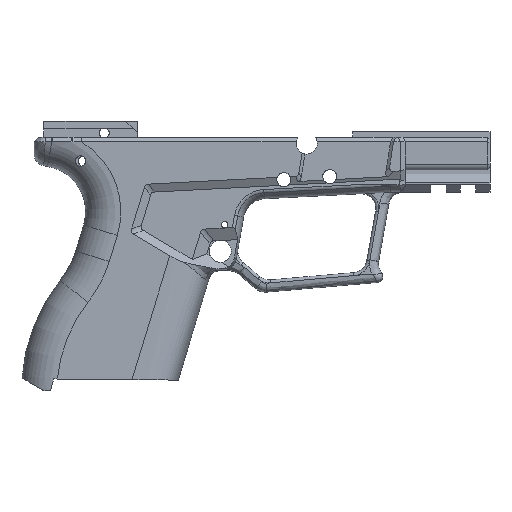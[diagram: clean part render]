
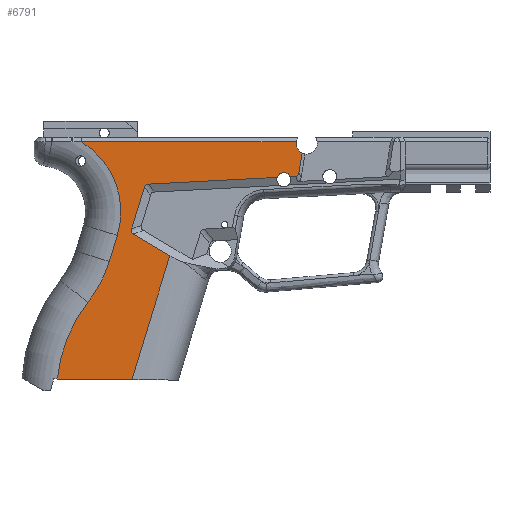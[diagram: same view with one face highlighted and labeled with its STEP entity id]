
A CAD part, left-side view. The second image highlights one B-rep face of the part: STEP entity #6791.
In plain terms, the highlighted planar face has unit normal (-1, 0, 0).
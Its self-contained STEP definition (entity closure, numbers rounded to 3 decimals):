
#60=ELLIPSE('',#6874,4.209,2.);
#64=ELLIPSE('',#6880,7.017,3.);
#66=ELLIPSE('',#6884,7.254,3.);
#545=PLANE('',#7359);
#892=FACE_OUTER_BOUND('',#1259,.T.);
#1259=EDGE_LOOP('',(#6368,#6369,#6370,#6371,#6372,#6373,#6374,#6375,#6376,
#6377,#6378,#6379,#6380,#6381,#6382,#6383,#6384,#6385));
#1333=CIRCLE('',#7027,2.4);
#1336=CIRCLE('',#7032,3.625);
#1445=CIRCLE('',#7334,48.221);
#1452=CIRCLE('',#7360,27.5);
#1453=CIRCLE('',#7361,42.);
#1534=LINE('',#9499,#2189);
#1575=LINE('',#9775,#2230);
#1579=LINE('',#9790,#2234);
#1584=LINE('',#9803,#2239);
#1587=LINE('',#9812,#2242);
#1589=LINE('',#9842,#2244);
#2095=LINE('',#15264,#2750);
#2109=LINE('',#15326,#2764);
#2110=LINE('',#15331,#2765);
#2111=LINE('',#15333,#2766);
#2189=VECTOR('',#7510,1000.);
#2230=VECTOR('',#7611,10.);
#2234=VECTOR('',#7625,10.);
#2239=VECTOR('',#7638,10.);
#2242=VECTOR('',#7649,10.);
#2244=VECTOR('',#7661,10.);
#2750=VECTOR('',#9075,10.);
#2764=VECTOR('',#9117,10.);
#2765=VECTOR('',#9122,10.);
#2766=VECTOR('',#9125,10.);
#2841=VERTEX_POINT('',#9497);
#2842=VERTEX_POINT('',#9498);
#2886=VERTEX_POINT('',#9772);
#2887=VERTEX_POINT('',#9774);
#2888=VERTEX_POINT('',#9778);
#2892=VERTEX_POINT('',#9787);
#2893=VERTEX_POINT('',#9789);
#2895=VERTEX_POINT('',#9795);
#2897=VERTEX_POINT('',#9800);
#2899=VERTEX_POINT('',#9807);
#2902=VERTEX_POINT('',#9836);
#3069=VERTEX_POINT('',#10879);
#3376=VERTEX_POINT('',#15017);
#3385=VERTEX_POINT('',#15198);
#3390=VERTEX_POINT('',#15231);
#3399=VERTEX_POINT('',#15262);
#3408=VERTEX_POINT('',#15328);
#3409=VERTEX_POINT('',#15330);
#3504=EDGE_CURVE('',#2841,#2842,#1534,.T.);
#3565=EDGE_CURVE('',#2887,#2886,#1575,.T.);
#3567=EDGE_CURVE('',#2887,#2888,#60,.T.);
#3572=EDGE_CURVE('',#2893,#2892,#1579,.T.);
#3575=EDGE_CURVE('',#2893,#2895,#64,.T.);
#3579=EDGE_CURVE('',#2897,#2895,#1584,.T.);
#3581=EDGE_CURVE('',#2897,#2899,#66,.T.);
#3584=EDGE_CURVE('',#2841,#2899,#1587,.T.);
#3592=EDGE_CURVE('',#2902,#2888,#1589,.T.);
#3823=EDGE_CURVE('',#2892,#2902,#1333,.F.);
#3830=EDGE_CURVE('',#2886,#3069,#1336,.T.);
#4375=EDGE_CURVE('',#3390,#3385,#1445,.T.);
#4391=EDGE_CURVE('',#3390,#3399,#2095,.F.);
#4411=EDGE_CURVE('',#3376,#3069,#2109,.T.);
#4412=EDGE_CURVE('',#3408,#3376,#1452,.T.);
#4413=EDGE_CURVE('',#3409,#3408,#2110,.T.);
#4414=EDGE_CURVE('',#3385,#3409,#1453,.T.);
#4415=EDGE_CURVE('',#2842,#3399,#2111,.T.);
#6368=ORIENTED_EDGE('',*,*,#4411,.F.);
#6369=ORIENTED_EDGE('',*,*,#4412,.F.);
#6370=ORIENTED_EDGE('',*,*,#4413,.F.);
#6371=ORIENTED_EDGE('',*,*,#4414,.F.);
#6372=ORIENTED_EDGE('',*,*,#4375,.F.);
#6373=ORIENTED_EDGE('',*,*,#4391,.T.);
#6374=ORIENTED_EDGE('',*,*,#4415,.F.);
#6375=ORIENTED_EDGE('',*,*,#3504,.F.);
#6376=ORIENTED_EDGE('',*,*,#3584,.T.);
#6377=ORIENTED_EDGE('',*,*,#3581,.F.);
#6378=ORIENTED_EDGE('',*,*,#3579,.T.);
#6379=ORIENTED_EDGE('',*,*,#3575,.F.);
#6380=ORIENTED_EDGE('',*,*,#3572,.T.);
#6381=ORIENTED_EDGE('',*,*,#3823,.T.);
#6382=ORIENTED_EDGE('',*,*,#3592,.T.);
#6383=ORIENTED_EDGE('',*,*,#3567,.F.);
#6384=ORIENTED_EDGE('',*,*,#3565,.T.);
#6385=ORIENTED_EDGE('',*,*,#3830,.T.);
#6791=ADVANCED_FACE('',(#892),#545,.F.);
#6874=AXIS2_PLACEMENT_3D('',#9779,#7615,#7616);
#6880=AXIS2_PLACEMENT_3D('',#9796,#7631,#7632);
#6884=AXIS2_PLACEMENT_3D('',#9808,#7643,#7644);
#7027=AXIS2_PLACEMENT_3D('',#10868,#8060,#8061);
#7032=AXIS2_PLACEMENT_3D('',#10881,#8073,#8074);
#7334=AXIS2_PLACEMENT_3D('',#15233,#9042,#9043);
#7359=AXIS2_PLACEMENT_3D('',#15327,#9118,#9119);
#7360=AXIS2_PLACEMENT_3D('',#15329,#9120,#9121);
#7361=AXIS2_PLACEMENT_3D('',#15332,#9123,#9124);
#7510=DIRECTION('',(0.,0.292,-0.956));
#7611=DIRECTION('',(0.,-0.156,0.988));
#7615=DIRECTION('center_axis',(1.,0.,0.));
#7616=DIRECTION('ref_axis',(0.,-0.402,-0.916));
#7625=DIRECTION('',(0.,-0.999,0.052));
#7631=DIRECTION('center_axis',(-1.,0.,0.));
#7632=DIRECTION('ref_axis',(0.,0.616,0.788));
#7638=DIRECTION('',(0.,-0.292,0.956));
#7643=DIRECTION('center_axis',(-1.,0.,0.));
#7644=DIRECTION('ref_axis',(0.,0.933,-0.36));
#7649=DIRECTION('',(0.,0.859,0.511));
#7661=DIRECTION('',(0.,-0.999,0.052));
#8060=DIRECTION('center_axis',(-1.,0.,0.));
#8061=DIRECTION('ref_axis',(0.,-1.,0.));
#8073=DIRECTION('center_axis',(1.,0.,0.));
#8074=DIRECTION('ref_axis',(0.,-1.,0.));
#9042=DIRECTION('center_axis',(1.,0.,0.));
#9043=DIRECTION('ref_axis',(0.,0.94,0.341));
#9075=DIRECTION('',(0.,0.999,0.035));
#9117=DIRECTION('',(0.,-1.,0.));
#9118=DIRECTION('center_axis',(1.,0.,0.));
#9119=DIRECTION('ref_axis',(0.,1.,0.));
#9120=DIRECTION('center_axis',(-1.,0.,0.));
#9121=DIRECTION('ref_axis',(0.,-0.853,0.522));
#9122=DIRECTION('',(0.,-0.292,0.956));
#9123=DIRECTION('center_axis',(-1.,0.,0.));
#9124=DIRECTION('ref_axis',(0.,-0.885,-0.465));
#9125=DIRECTION('',(0.,1.,0.009));
#9497=CARTESIAN_POINT('',(-15.125,38.555,47.5));
#9498=CARTESIAN_POINT('',(-15.125,51.377,5.562));
#9499=CARTESIAN_POINT('',(-15.125,40.084,42.5));
#9772=CARTESIAN_POINT('',(-15.125,-6.167,82.239));
#9774=CARTESIAN_POINT('',(-15.125,-5.121,75.638));
#9775=CARTESIAN_POINT('',(-15.125,-2.368,58.256));
#9778=CARTESIAN_POINT('',(-15.125,-4.013,74.322));
#9779=CARTESIAN_POINT('Origin',(-15.125,-2.672,78.257));
#9787=CARTESIAN_POINT('',(-15.125,2.282,73.992));
#9789=CARTESIAN_POINT('',(-15.125,45.806,71.711));
#9790=CARTESIAN_POINT('',(-15.125,-21.047,75.215));
#9795=CARTESIAN_POINT('',(-15.125,47.162,70.652));
#9796=CARTESIAN_POINT('Origin',(-15.125,42.346,65.884));
#9800=CARTESIAN_POINT('',(-15.125,51.481,56.524));
#9803=CARTESIAN_POINT('',(-15.125,48.616,65.895));
#9807=CARTESIAN_POINT('',(-15.125,50.814,54.797));
#9808=CARTESIAN_POINT('Origin',(-15.125,44.711,58.147));
#9812=CARTESIAN_POINT('',(-15.125,31.265,43.161));
#9836=CARTESIAN_POINT('',(-15.125,-2.192,74.227));
#9842=CARTESIAN_POINT('',(-15.125,-21.047,75.215));
#10868=CARTESIAN_POINT('Origin',(-15.125,0.,73.25));
#10879=CARTESIAN_POINT('',(-15.125,-4.16,86.));
#10881=CARTESIAN_POINT('Origin',(-15.125,-7.75,85.5));
#15017=CARTESIAN_POINT('',(-15.125,68.451,86.));
#15198=CARTESIAN_POINT('',(-15.125,66.274,31.751));
#15231=CARTESIAN_POINT('',(-15.125,76.553,5.782));
#15233=CARTESIAN_POINT('Origin',(-15.125,28.499,1.78));
#15262=CARTESIAN_POINT('',(-15.125,76.531,5.782));
#15264=CARTESIAN_POINT('',(-15.125,7.252,3.362));
#15326=CARTESIAN_POINT('',(-15.125,43.3,86.));
#15327=CARTESIAN_POINT('Origin',(-15.125,2.101,45.375));
#15328=CARTESIAN_POINT('',(-15.125,56.317,54.388));
#15329=CARTESIAN_POINT('Origin',(-15.125,82.616,62.429));
#15330=CARTESIAN_POINT('',(-15.125,59.011,45.577));
#15331=CARTESIAN_POINT('',(-15.125,57.524,50.441));
#15332=CARTESIAN_POINT('Origin',(-15.125,99.176,57.856));
#15333=CARTESIAN_POINT('',(-15.125,6.135,5.167));
